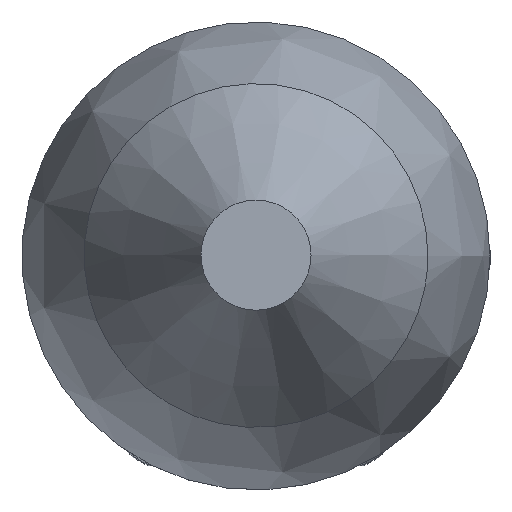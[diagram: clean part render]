
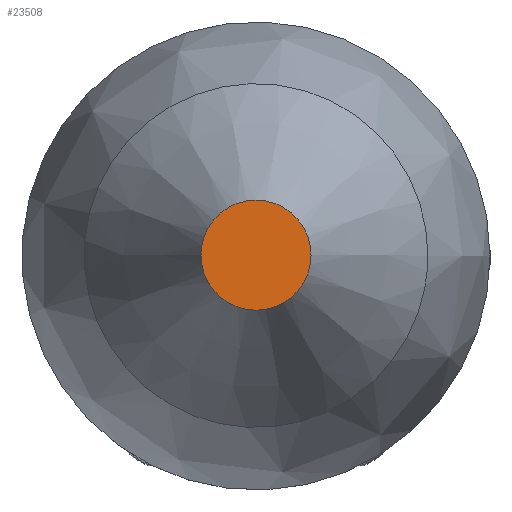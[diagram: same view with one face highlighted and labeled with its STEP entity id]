
A CAD part, top view. The second image highlights one B-rep face of the part: STEP entity #23508.
In plain terms, the highlighted planar face has unit normal (0, 0, 1).
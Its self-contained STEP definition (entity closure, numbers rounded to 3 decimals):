
#23409 = CONICAL_SURFACE('',#23410,17.,0.48);
#23410 = AXIS2_PLACEMENT_3D('',#23411,#23412,#23413);
#23411 = CARTESIAN_POINT('',(0.,0.,177.));
#23412 = DIRECTION('',(-0.,-0.,-1.));
#23413 = DIRECTION('',(1.,0.,0.));
#23458 = VERTEX_POINT('',#23459);
#23459 = CARTESIAN_POINT('',(4.,0.,202.));
#23480 = EDGE_CURVE('',#23458,#23458,#23481,.T.);
#23481 = SURFACE_CURVE('',#23482,(#23487,#23494),.PCURVE_S1.);
#23482 = CIRCLE('',#23483,4.);
#23483 = AXIS2_PLACEMENT_3D('',#23484,#23485,#23486);
#23484 = CARTESIAN_POINT('',(0.,0.,202.));
#23485 = DIRECTION('',(0.,0.,1.));
#23486 = DIRECTION('',(1.,0.,0.));
#23487 = PCURVE('',#23409,#23488);
#23488 = DEFINITIONAL_REPRESENTATION('',(#23489),#23493);
#23489 = LINE('',#23490,#23491);
#23490 = CARTESIAN_POINT('',(-0.,-25.));
#23491 = VECTOR('',#23492,1.);
#23492 = DIRECTION('',(-1.,-0.));
#23493 = ( GEOMETRIC_REPRESENTATION_CONTEXT(2) 
PARAMETRIC_REPRESENTATION_CONTEXT() REPRESENTATION_CONTEXT('2D SPACE',''
  ) );
#23494 = PCURVE('',#23495,#23500);
#23495 = PLANE('',#23496);
#23496 = AXIS2_PLACEMENT_3D('',#23497,#23498,#23499);
#23497 = CARTESIAN_POINT('',(0.,0.,202.));
#23498 = DIRECTION('',(0.,0.,1.));
#23499 = DIRECTION('',(1.,0.,0.));
#23500 = DEFINITIONAL_REPRESENTATION('',(#23501),#23505);
#23501 = CIRCLE('',#23502,4.);
#23502 = AXIS2_PLACEMENT_2D('',#23503,#23504);
#23503 = CARTESIAN_POINT('',(0.,0.));
#23504 = DIRECTION('',(1.,0.));
#23505 = ( GEOMETRIC_REPRESENTATION_CONTEXT(2) 
PARAMETRIC_REPRESENTATION_CONTEXT() REPRESENTATION_CONTEXT('2D SPACE',''
  ) );
#23508 = ADVANCED_FACE('',(#23509),#23495,.T.);
#23509 = FACE_BOUND('',#23510,.T.);
#23510 = EDGE_LOOP('',(#23511));
#23511 = ORIENTED_EDGE('',*,*,#23480,.T.);
